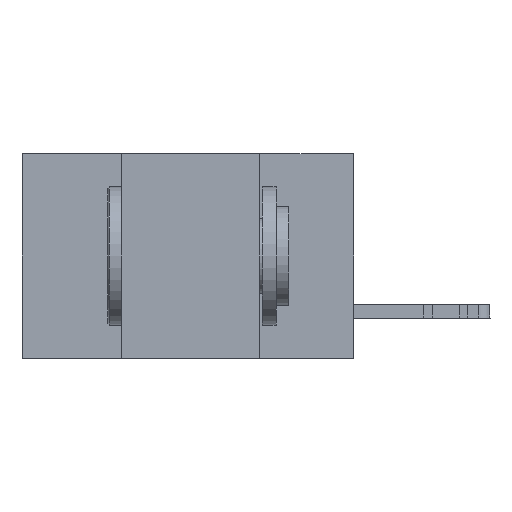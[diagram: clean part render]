
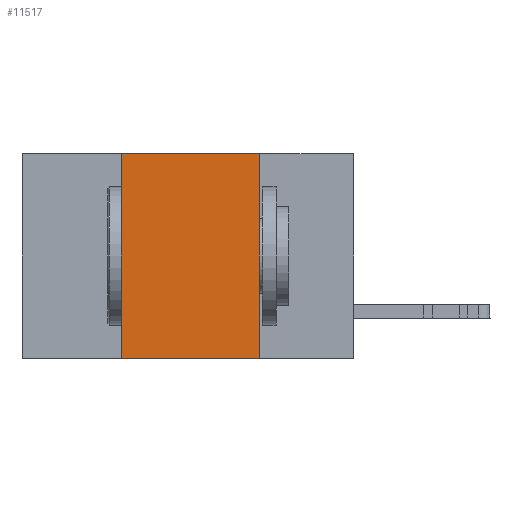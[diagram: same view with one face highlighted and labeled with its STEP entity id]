
A CAD part, left-side view. The second image highlights one B-rep face of the part: STEP entity #11517.
In plain terms, the highlighted planar face has unit normal (-1, 0, 0).
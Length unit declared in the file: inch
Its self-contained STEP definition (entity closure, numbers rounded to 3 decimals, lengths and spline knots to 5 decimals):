
#339 = VERTEX_POINT ( 'NONE', #33344 ) ;
#872 = DIRECTION ( 'NONE',  ( 0., 0., 1. ) ) ;
#2122 = VECTOR ( 'NONE', #872, 39.37008 ) ;
#4495 = LINE ( 'NONE', #16719, #19418 ) ;
#6153 = VERTEX_POINT ( 'NONE', #26678 ) ;
#7276 = DIRECTION ( 'NONE',  ( 0., 0., -1. ) ) ;
#7528 = EDGE_CURVE ( 'NONE', #15026, #35042, #31620, .T. ) ;
#8415 = CARTESIAN_POINT ( 'NONE',  ( 0., 0.17, -0.37 ) ) ;
#10454 = LINE ( 'NONE', #35359, #2122 ) ;
#11517 = ADVANCED_FACE ( 'NONE', ( #18442 ), #33212, .F. ) ;
#13668 = EDGE_LOOP ( 'NONE', ( #19212, #16765, #27751, #15732 ) ) ;
#15026 = VERTEX_POINT ( 'NONE', #36902 ) ;
#15732 = ORIENTED_EDGE ( 'NONE', *, *, #7528, .T. ) ;
#16719 = CARTESIAN_POINT ( 'NONE',  ( 0., 0.17, 0. ) ) ;
#16765 = ORIENTED_EDGE ( 'NONE', *, *, #29542, .F. ) ;
#18442 = FACE_OUTER_BOUND ( 'NONE', #13668, .T. ) ;
#19212 = ORIENTED_EDGE ( 'NONE', *, *, #34897, .F. ) ;
#19364 = DIRECTION ( 'NONE',  ( 1., 0., 0. ) ) ;
#19418 = VECTOR ( 'NONE', #7276, 39.37008 ) ;
#20569 = EDGE_CURVE ( 'NONE', #15026, #339, #10454, .T. ) ;
#23707 = DIRECTION ( 'NONE',  ( 0., -1., 0. ) ) ;
#24398 = DIRECTION ( 'NONE',  ( 0., -1., 0. ) ) ;
#26678 = CARTESIAN_POINT ( 'NONE',  ( 0., 0.17, 0. ) ) ;
#27751 = ORIENTED_EDGE ( 'NONE', *, *, #20569, .F. ) ;
#29205 = CARTESIAN_POINT ( 'NONE',  ( 0., 0.6, 0. ) ) ;
#29542 = EDGE_CURVE ( 'NONE', #339, #6153, #34656, .T. ) ;
#31620 = LINE ( 'NONE', #34302, #38946 ) ;
#33165 = VECTOR ( 'NONE', #23707, 39.37008 ) ;
#33212 = PLANE ( 'NONE',  #35582 ) ;
#33344 = CARTESIAN_POINT ( 'NONE',  ( 0., 0.42, 0. ) ) ;
#34302 = CARTESIAN_POINT ( 'NONE',  ( 0., 0.6, -0.37 ) ) ;
#34656 = LINE ( 'NONE', #29205, #33165 ) ;
#34897 = EDGE_CURVE ( 'NONE', #6153, #35042, #4495, .T. ) ;
#34973 = CARTESIAN_POINT ( 'NONE',  ( 0., 0.6, 0. ) ) ;
#35042 = VERTEX_POINT ( 'NONE', #8415 ) ;
#35359 = CARTESIAN_POINT ( 'NONE',  ( 0., 0.42, 0. ) ) ;
#35582 = AXIS2_PLACEMENT_3D ( 'NONE', #34973, #19364, #35882 ) ;
#35882 = DIRECTION ( 'NONE',  ( 0., 0., -1. ) ) ;
#36902 = CARTESIAN_POINT ( 'NONE',  ( 0., 0.42, -0.37 ) ) ;
#38946 = VECTOR ( 'NONE', #24398, 39.37008 ) ;
